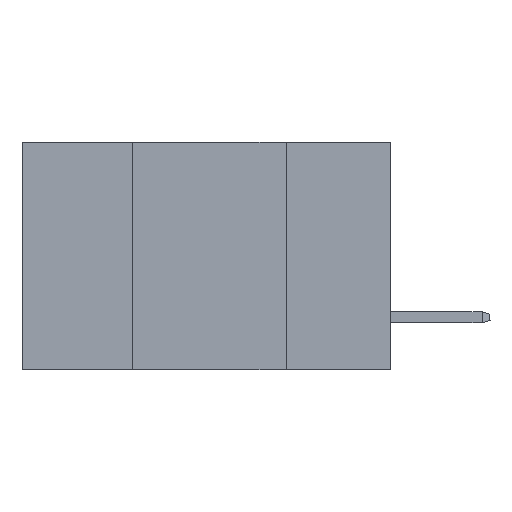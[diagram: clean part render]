
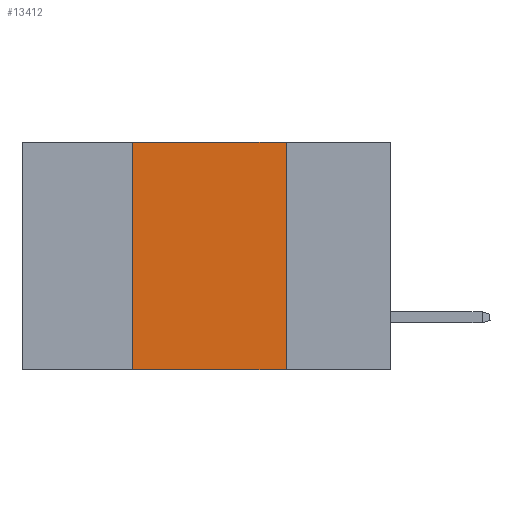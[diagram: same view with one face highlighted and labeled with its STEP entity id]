
A CAD part, left-side view. The second image highlights one B-rep face of the part: STEP entity #13412.
In plain terms, the highlighted planar face has unit normal (-1, 0, 0).
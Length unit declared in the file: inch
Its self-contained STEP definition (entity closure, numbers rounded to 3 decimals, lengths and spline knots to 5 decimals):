
#339 = ORIENTED_EDGE ( 'NONE', *, *, #18302, .F. ) ;
#765 = CARTESIAN_POINT ( 'NONE',  ( 0., 0.6, -0.37 ) ) ;
#1282 = CARTESIAN_POINT ( 'NONE',  ( 0., 0.17, 0. ) ) ;
#1565 = DIRECTION ( 'NONE',  ( 0., 0., -1. ) ) ;
#1936 = EDGE_CURVE ( 'NONE', #15243, #12061, #11101, .T. ) ;
#3988 = LINE ( 'NONE', #765, #11900 ) ;
#4850 = VECTOR ( 'NONE', #15634, 39.37008 ) ;
#5212 = ORIENTED_EDGE ( 'NONE', *, *, #1936, .F. ) ;
#6019 = VERTEX_POINT ( 'NONE', #19620 ) ;
#6456 = VECTOR ( 'NONE', #1565, 39.37008 ) ;
#6904 = VECTOR ( 'NONE', #16181, 39.37008 ) ;
#6918 = EDGE_CURVE ( 'NONE', #15243, #6019, #3988, .T. ) ;
#8158 = FACE_OUTER_BOUND ( 'NONE', #12248, .T. ) ;
#9046 = LINE ( 'NONE', #12955, #4850 ) ;
#9113 = DIRECTION ( 'NONE',  ( 0., 0., -1. ) ) ;
#11101 = LINE ( 'NONE', #16041, #6904 ) ;
#11883 = DIRECTION ( 'NONE',  ( 0., -1., 0. ) ) ;
#11900 = VECTOR ( 'NONE', #11883, 39.37008 ) ;
#12061 = VERTEX_POINT ( 'NONE', #13583 ) ;
#12248 = EDGE_LOOP ( 'NONE', ( #20550, #339, #5212, #20566 ) ) ;
#12713 = EDGE_CURVE ( 'NONE', #18724, #6019, #19163, .T. ) ;
#12942 = CARTESIAN_POINT ( 'NONE',  ( 0., 0.42, -0.37 ) ) ;
#12955 = CARTESIAN_POINT ( 'NONE',  ( 0., 0.6, 0. ) ) ;
#13412 = ADVANCED_FACE ( 'NONE', ( #8158 ), #18714, .F. ) ;
#13583 = CARTESIAN_POINT ( 'NONE',  ( 0., 0.42, 0. ) ) ;
#15243 = VERTEX_POINT ( 'NONE', #12942 ) ;
#15577 = DIRECTION ( 'NONE',  ( 1., 0., 0. ) ) ;
#15634 = DIRECTION ( 'NONE',  ( 0., -1., 0. ) ) ;
#15652 = CARTESIAN_POINT ( 'NONE',  ( 0., 0.6, 0. ) ) ;
#15716 = AXIS2_PLACEMENT_3D ( 'NONE', #15652, #15577, #9113 ) ;
#16041 = CARTESIAN_POINT ( 'NONE',  ( 0., 0.42, 0. ) ) ;
#16181 = DIRECTION ( 'NONE',  ( 0., 0., 1. ) ) ;
#16270 = CARTESIAN_POINT ( 'NONE',  ( 0., 0.17, 0. ) ) ;
#18302 = EDGE_CURVE ( 'NONE', #12061, #18724, #9046, .T. ) ;
#18714 = PLANE ( 'NONE',  #15716 ) ;
#18724 = VERTEX_POINT ( 'NONE', #16270 ) ;
#19163 = LINE ( 'NONE', #1282, #6456 ) ;
#19620 = CARTESIAN_POINT ( 'NONE',  ( 0., 0.17, -0.37 ) ) ;
#20550 = ORIENTED_EDGE ( 'NONE', *, *, #12713, .F. ) ;
#20566 = ORIENTED_EDGE ( 'NONE', *, *, #6918, .T. ) ;
